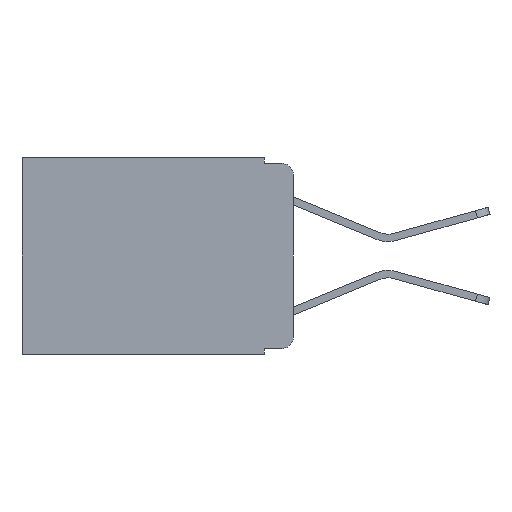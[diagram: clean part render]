
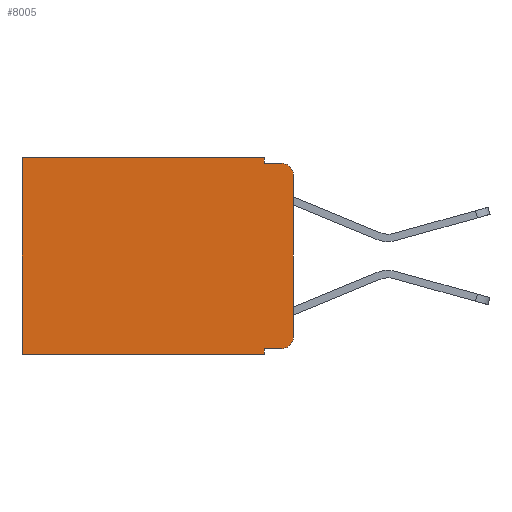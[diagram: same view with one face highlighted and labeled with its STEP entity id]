
A CAD part, left-side view. The second image highlights one B-rep face of the part: STEP entity #8005.
In plain terms, the highlighted planar face has unit normal (-1, 0, 0).
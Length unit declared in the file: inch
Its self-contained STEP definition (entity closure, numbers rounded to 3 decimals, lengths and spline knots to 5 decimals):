
#79 = VERTEX_POINT ( 'NONE', #8406 ) ;
#172 = FACE_OUTER_BOUND ( 'NONE', #11896, .T. ) ;
#284 = EDGE_CURVE ( 'NONE', #6735, #79, #7785, .T. ) ;
#413 = CARTESIAN_POINT ( 'NONE',  ( 0.298, 0.051, -0.343 ) ) ;
#471 = DIRECTION ( 'NONE',  ( 0., 0., -1. ) ) ;
#481 = EDGE_CURVE ( 'NONE', #5704, #6546, #4244, .T. ) ;
#624 = EDGE_CURVE ( 'NONE', #7927, #7319, #11106, .T. ) ;
#631 = EDGE_CURVE ( 'NONE', #7927, #1724, #6330, .T. ) ;
#652 = EDGE_CURVE ( 'NONE', #8203, #1724, #11622, .T. ) ;
#654 = EDGE_CURVE ( 'NONE', #6735, #8203, #10831, .T. ) ;
#657 = EDGE_CURVE ( 'NONE', #79, #6546, #1002, .T. ) ;
#673 = EDGE_CURVE ( 'NONE', #11429, #5704, #10286, .T. ) ;
#678 = VECTOR ( 'NONE', #12077, 39.37008 ) ;
#691 = EDGE_CURVE ( 'NONE', #11429, #9587, #2813, .T. ) ;
#706 = EDGE_CURVE ( 'NONE', #9587, #7319, #12019, .T. ) ;
#832 = CARTESIAN_POINT ( 'NONE',  ( 0.298, 0.473, -0.343 ) ) ;
#891 = CARTESIAN_POINT ( 'NONE',  ( 0.298, 0.051, -0.01 ) ) ;
#1002 = LINE ( 'NONE', #3275, #678 ) ;
#1236 = AXIS2_PLACEMENT_3D ( 'NONE', #9158, #9551, #1988 ) ;
#1323 = CARTESIAN_POINT ( 'NONE',  ( 0.298, 0., 0. ) ) ;
#1411 = CARTESIAN_POINT ( 'NONE',  ( 0.298, 0., 0. ) ) ;
#1724 = VERTEX_POINT ( 'NONE', #6037 ) ;
#1988 = DIRECTION ( 'NONE',  ( 0., 0., -1. ) ) ;
#2199 = CARTESIAN_POINT ( 'NONE',  ( 0.298, 0.051, -0.01 ) ) ;
#2272 = ORIENTED_EDGE ( 'NONE', *, *, #652, .F. ) ;
#2460 = VECTOR ( 'NONE', #11273, 39.37008 ) ;
#2752 = DIRECTION ( 'NONE',  ( 0., 0., -1. ) ) ;
#2813 = LINE ( 'NONE', #8287, #2460 ) ;
#2876 = CARTESIAN_POINT ( 'NONE',  ( 0.298, 0.051, -0.333 ) ) ;
#3275 = CARTESIAN_POINT ( 'NONE',  ( 0.298, 0.473, 0. ) ) ;
#3812 = CARTESIAN_POINT ( 'NONE',  ( 0.298, 0., -0.313 ) ) ;
#3950 = VECTOR ( 'NONE', #6807, 39.37008 ) ;
#4085 = CARTESIAN_POINT ( 'NONE',  ( 0.298, 0.051, 0. ) ) ;
#4087 = VECTOR ( 'NONE', #10466, 39.37008 ) ;
#4224 = ORIENTED_EDGE ( 'NONE', *, *, #481, .F. ) ;
#4244 = LINE ( 'NONE', #8756, #3950 ) ;
#4356 = AXIS2_PLACEMENT_3D ( 'NONE', #9484, #8200, #2752 ) ;
#4539 = ORIENTED_EDGE ( 'NONE', *, *, #691, .T. ) ;
#4715 = PLANE ( 'NONE',  #10599 ) ;
#5004 = VECTOR ( 'NONE', #10858, 39.37008 ) ;
#5141 = DIRECTION ( 'NONE',  ( 0., 0., -1. ) ) ;
#5436 = VECTOR ( 'NONE', #8418, 39.37008 ) ;
#5675 = DIRECTION ( 'NONE',  ( 1., 0., 0. ) ) ;
#5704 = VERTEX_POINT ( 'NONE', #413 ) ;
#5921 = CARTESIAN_POINT ( 'NONE',  ( 0.298, 0.02, -0.333 ) ) ;
#6032 = VECTOR ( 'NONE', #471, 39.37008 ) ;
#6037 = CARTESIAN_POINT ( 'NONE',  ( 0.298, 0.02, -0.01 ) ) ;
#6167 = ORIENTED_EDGE ( 'NONE', *, *, #284, .T. ) ;
#6330 = CIRCLE ( 'NONE', #1236, 0.02 ) ;
#6451 = CARTESIAN_POINT ( 'NONE',  ( 0.298, 0., -0.03 ) ) ;
#6546 = VERTEX_POINT ( 'NONE', #832 ) ;
#6735 = VERTEX_POINT ( 'NONE', #4085 ) ;
#6807 = DIRECTION ( 'NONE',  ( 0., 1., 0. ) ) ;
#7319 = VERTEX_POINT ( 'NONE', #3812 ) ;
#7785 = LINE ( 'NONE', #1411, #5004 ) ;
#7927 = VERTEX_POINT ( 'NONE', #6451 ) ;
#8005 = ADVANCED_FACE ( 'NONE', ( #172 ), #4715, .F. ) ;
#8188 = ORIENTED_EDGE ( 'NONE', *, *, #706, .T. ) ;
#8200 = DIRECTION ( 'NONE',  ( -1., 0., 0. ) ) ;
#8203 = VERTEX_POINT ( 'NONE', #891 ) ;
#8211 = CARTESIAN_POINT ( 'NONE',  ( 0.298, 0.051, 0. ) ) ;
#8287 = CARTESIAN_POINT ( 'NONE',  ( 0.298, 0.051, -0.333 ) ) ;
#8406 = CARTESIAN_POINT ( 'NONE',  ( 0.298, 0.473, 0. ) ) ;
#8418 = DIRECTION ( 'NONE',  ( 0., 0., -1. ) ) ;
#8756 = CARTESIAN_POINT ( 'NONE',  ( 0.298, 0., -0.343 ) ) ;
#8774 = ORIENTED_EDGE ( 'NONE', *, *, #631, .T. ) ;
#8792 = VECTOR ( 'NONE', #5141, 39.37008 ) ;
#9050 = ORIENTED_EDGE ( 'NONE', *, *, #624, .F. ) ;
#9158 = CARTESIAN_POINT ( 'NONE',  ( 0.298, 0.02, -0.03 ) ) ;
#9345 = ORIENTED_EDGE ( 'NONE', *, *, #654, .F. ) ;
#9484 = CARTESIAN_POINT ( 'NONE',  ( 0.298, 0.02, -0.313 ) ) ;
#9551 = DIRECTION ( 'NONE',  ( -1., 0., 0. ) ) ;
#9587 = VERTEX_POINT ( 'NONE', #5921 ) ;
#9878 = ORIENTED_EDGE ( 'NONE', *, *, #657, .T. ) ;
#10097 = CARTESIAN_POINT ( 'NONE',  ( 0.298, 0.051, 0. ) ) ;
#10206 = CARTESIAN_POINT ( 'NONE',  ( 0.298, 0., 0. ) ) ;
#10286 = LINE ( 'NONE', #8211, #5436 ) ;
#10466 = DIRECTION ( 'NONE',  ( 0., -1., 0. ) ) ;
#10599 = AXIS2_PLACEMENT_3D ( 'NONE', #10206, #5675, #11922 ) ;
#10831 = LINE ( 'NONE', #10097, #6032 ) ;
#10858 = DIRECTION ( 'NONE',  ( 0., 1., 0. ) ) ;
#10953 = ORIENTED_EDGE ( 'NONE', *, *, #673, .F. ) ;
#11106 = LINE ( 'NONE', #1323, #8792 ) ;
#11273 = DIRECTION ( 'NONE',  ( 0., -1., 0. ) ) ;
#11429 = VERTEX_POINT ( 'NONE', #2876 ) ;
#11622 = LINE ( 'NONE', #2199, #4087 ) ;
#11896 = EDGE_LOOP ( 'NONE', ( #9050, #8774, #2272, #9345, #6167, #9878, #4224, #10953, #4539, #8188 ) ) ;
#11922 = DIRECTION ( 'NONE',  ( 0., 0., -1. ) ) ;
#12019 = CIRCLE ( 'NONE', #4356, 0.02 ) ;
#12077 = DIRECTION ( 'NONE',  ( 0., 0., -1. ) ) ;
